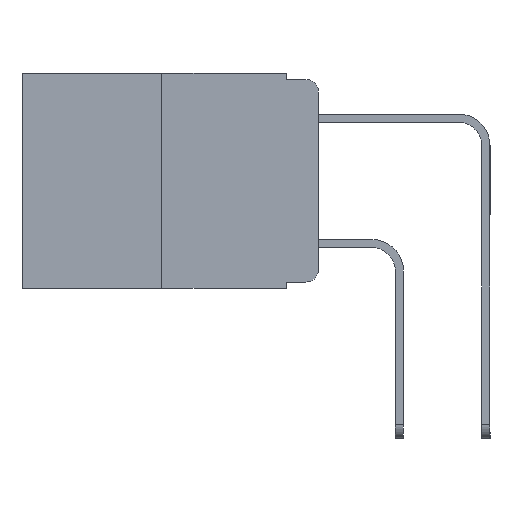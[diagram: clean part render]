
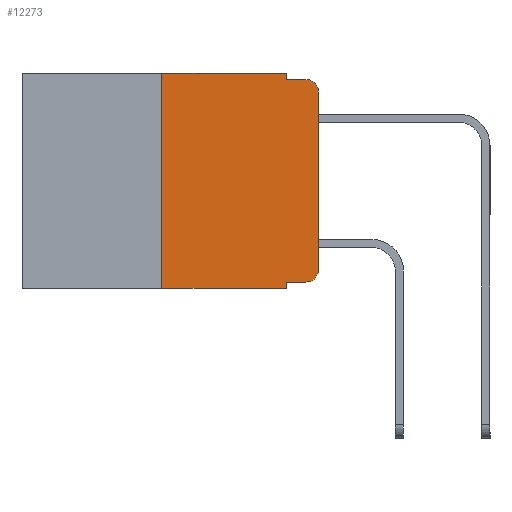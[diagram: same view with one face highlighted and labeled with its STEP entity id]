
A CAD part, left-side view. The second image highlights one B-rep face of the part: STEP entity #12273.
In plain terms, the highlighted planar face has unit normal (-1, 0, 0).
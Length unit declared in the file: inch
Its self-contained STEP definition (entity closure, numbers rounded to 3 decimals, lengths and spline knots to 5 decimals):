
#181 = CARTESIAN_POINT ( 'NONE',  ( 0., 0.473, 0. ) ) ;
#253 = EDGE_CURVE ( 'NONE', #17299, #5793, #2932, .T. ) ;
#259 = DIRECTION ( 'NONE',  ( 0., -1., 0. ) ) ;
#267 = ORIENTED_EDGE ( 'NONE', *, *, #253, .F. ) ;
#353 = ORIENTED_EDGE ( 'NONE', *, *, #13177, .F. ) ;
#817 = ORIENTED_EDGE ( 'NONE', *, *, #18993, .F. ) ;
#879 = ORIENTED_EDGE ( 'NONE', *, *, #10544, .T. ) ;
#1281 = VERTEX_POINT ( 'NONE', #3423 ) ;
#1501 = CARTESIAN_POINT ( 'NONE',  ( 0., 0., -0.313 ) ) ;
#1607 = ORIENTED_EDGE ( 'NONE', *, *, #17988, .F. ) ;
#1740 = ORIENTED_EDGE ( 'NONE', *, *, #14826, .T. ) ;
#1985 = ORIENTED_EDGE ( 'NONE', *, *, #13796, .T. ) ;
#1994 = DIRECTION ( 'NONE',  ( 0., -1., 0. ) ) ;
#2409 = CARTESIAN_POINT ( 'NONE',  ( 0., 0.02, -0.333 ) ) ;
#2446 = LINE ( 'NONE', #4784, #10643 ) ;
#2480 = CIRCLE ( 'NONE', #13325, 0.02 ) ;
#2563 = EDGE_CURVE ( 'NONE', #5793, #5148, #16128, .T. ) ;
#2932 = LINE ( 'NONE', #13843, #11601 ) ;
#2976 = CARTESIAN_POINT ( 'NONE',  ( 0., 0.473, 0. ) ) ;
#3224 = CARTESIAN_POINT ( 'NONE',  ( 0., 0.051, -0.333 ) ) ;
#3343 = VECTOR ( 'NONE', #11557, 39.37008 ) ;
#3423 = CARTESIAN_POINT ( 'NONE',  ( 0., 0.25, 0. ) ) ;
#3453 = VERTEX_POINT ( 'NONE', #1501 ) ;
#3758 = CARTESIAN_POINT ( 'NONE',  ( 0., 0., 0. ) ) ;
#4476 = EDGE_LOOP ( 'NONE', ( #17640, #17007, #15457, #267, #353, #817, #879, #1607, #1740, #1985 ) ) ;
#4675 = DIRECTION ( 'NONE',  ( 0., 0., -1. ) ) ;
#4784 = CARTESIAN_POINT ( 'NONE',  ( 0., 0.051, 0. ) ) ;
#5148 = VERTEX_POINT ( 'NONE', #12925 ) ;
#5348 = DIRECTION ( 'NONE',  ( -1., 0., 0. ) ) ;
#5793 = VERTEX_POINT ( 'NONE', #7591 ) ;
#5936 = EDGE_CURVE ( 'NONE', #6925, #5148, #2480, .T. ) ;
#6281 = DIRECTION ( 'NONE',  ( 0., 0., -1. ) ) ;
#6301 = LINE ( 'NONE', #181, #17905 ) ;
#6335 = VECTOR ( 'NONE', #12198, 39.37008 ) ;
#6470 = DIRECTION ( 'NONE',  ( 0., 0., -1. ) ) ;
#6874 = CARTESIAN_POINT ( 'NONE',  ( 0., 0., -0.03 ) ) ;
#6925 = VERTEX_POINT ( 'NONE', #6874 ) ;
#7047 = EDGE_CURVE ( 'NONE', #3453, #6925, #20463, .T. ) ;
#7155 = DIRECTION ( 'NONE',  ( 0., 0., 1. ) ) ;
#7376 = FACE_OUTER_BOUND ( 'NONE', #4476, .T. ) ;
#7591 = CARTESIAN_POINT ( 'NONE',  ( 0., 0.051, -0.01 ) ) ;
#7944 = VERTEX_POINT ( 'NONE', #12386 ) ;
#8060 = VECTOR ( 'NONE', #7155, 39.37008 ) ;
#8807 = CARTESIAN_POINT ( 'NONE',  ( 0., 0.051, -0.01 ) ) ;
#8879 = DIRECTION ( 'NONE',  ( -1., 0., 0. ) ) ;
#8938 = VERTEX_POINT ( 'NONE', #2409 ) ;
#10102 = LINE ( 'NONE', #12339, #6335 ) ;
#10195 = CARTESIAN_POINT ( 'NONE',  ( 0., 0.051, -0.333 ) ) ;
#10544 = EDGE_CURVE ( 'NONE', #7944, #11562, #10850, .T. ) ;
#10643 = VECTOR ( 'NONE', #6470, 39.37008 ) ;
#10850 = LINE ( 'NONE', #13773, #19107 ) ;
#11420 = AXIS2_PLACEMENT_3D ( 'NONE', #2976, #14262, #4675 ) ;
#11469 = VECTOR ( 'NONE', #1994, 39.37008 ) ;
#11557 = DIRECTION ( 'NONE',  ( 0., -1., 0. ) ) ;
#11562 = VERTEX_POINT ( 'NONE', #13532 ) ;
#11601 = VECTOR ( 'NONE', #6281, 39.37008 ) ;
#11747 = CARTESIAN_POINT ( 'NONE',  ( 0., 0.051, 0. ) ) ;
#11852 = AXIS2_PLACEMENT_3D ( 'NONE', #14872, #5348, #16439 ) ;
#11960 = LINE ( 'NONE', #10195, #11469 ) ;
#12198 = DIRECTION ( 'NONE',  ( 0., 0., 1. ) ) ;
#12273 = ADVANCED_FACE ( 'NONE', ( #7376 ), #12710, .F. ) ;
#12339 = CARTESIAN_POINT ( 'NONE',  ( 0., 0.25, 0. ) ) ;
#12386 = CARTESIAN_POINT ( 'NONE',  ( 0., 0.25, -0.343 ) ) ;
#12710 = PLANE ( 'NONE',  #11420 ) ;
#12925 = CARTESIAN_POINT ( 'NONE',  ( 0., 0.02, -0.01 ) ) ;
#13177 = EDGE_CURVE ( 'NONE', #1281, #17299, #6301, .T. ) ;
#13325 = AXIS2_PLACEMENT_3D ( 'NONE', #19428, #8879, #15913 ) ;
#13532 = CARTESIAN_POINT ( 'NONE',  ( 0., 0.051, -0.343 ) ) ;
#13773 = CARTESIAN_POINT ( 'NONE',  ( 0., 0.473, -0.343 ) ) ;
#13796 = EDGE_CURVE ( 'NONE', #8938, #3453, #19050, .T. ) ;
#13843 = CARTESIAN_POINT ( 'NONE',  ( 0., 0.051, 0. ) ) ;
#14262 = DIRECTION ( 'NONE',  ( 1., 0., 0. ) ) ;
#14826 = EDGE_CURVE ( 'NONE', #20644, #8938, #11960, .T. ) ;
#14872 = CARTESIAN_POINT ( 'NONE',  ( 0., 0.02, -0.313 ) ) ;
#15326 = DIRECTION ( 'NONE',  ( 0., -1., 0. ) ) ;
#15457 = ORIENTED_EDGE ( 'NONE', *, *, #2563, .F. ) ;
#15913 = DIRECTION ( 'NONE',  ( 0., 0., -1. ) ) ;
#16128 = LINE ( 'NONE', #8807, #3343 ) ;
#16439 = DIRECTION ( 'NONE',  ( 0., 0., -1. ) ) ;
#17007 = ORIENTED_EDGE ( 'NONE', *, *, #5936, .T. ) ;
#17299 = VERTEX_POINT ( 'NONE', #11747 ) ;
#17640 = ORIENTED_EDGE ( 'NONE', *, *, #7047, .T. ) ;
#17905 = VECTOR ( 'NONE', #259, 39.37008 ) ;
#17988 = EDGE_CURVE ( 'NONE', #20644, #11562, #2446, .T. ) ;
#18993 = EDGE_CURVE ( 'NONE', #7944, #1281, #10102, .T. ) ;
#19050 = CIRCLE ( 'NONE', #11852, 0.02 ) ;
#19107 = VECTOR ( 'NONE', #15326, 39.37008 ) ;
#19428 = CARTESIAN_POINT ( 'NONE',  ( 0., 0.02, -0.03 ) ) ;
#20463 = LINE ( 'NONE', #3758, #8060 ) ;
#20644 = VERTEX_POINT ( 'NONE', #3224 ) ;
